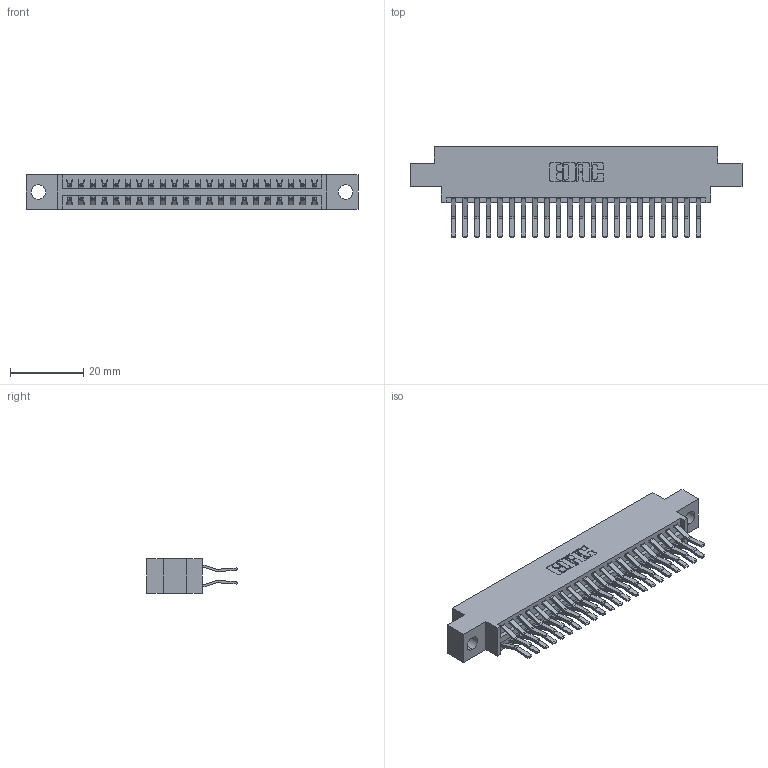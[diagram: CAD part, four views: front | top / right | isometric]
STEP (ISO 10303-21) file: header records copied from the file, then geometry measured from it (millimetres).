
FILE_DESCRIPTION (( 'STEP AP203' ), '1' );
FILE_NAME ('346-044-560-804.STEP', '2022-05-20T08:39:11', ( '' ), ( '' ), 'SwSTEP 2.0', 'SolidWorks 2020', '' );
FILE_SCHEMA (( 'CONFIG_CONTROL_DESIGN' ));
Length unit declared in the file: inch
Products named in the file (3): 346 Part_0.170 Offset - 0.156 Dia-TH; 346-044-560-804; 345-292-001_560 Tail
Assembly tree (45 placements, depth 2):
  346-044-560-804
    346 Part_0.170 Offset - 0.156 Dia-TH
    345-292-001_560 Tail  x44
Bounding box: 90.42 x 24.78 x 9.4 mm (x, y, z)
Volume: 8690 mm3; surface area: 12427.6 mm2
Topology: 45 solids, 45 shells, 2516 faces, 7461 edges, 4914 vertices
Faces by surface type: plane 1634, cylinder 882
Entity records: 17689 total; most frequent: CARTESIAN_POINT 2950, ORIENTED_EDGE 2882, DIRECTION 2653, EDGE_CURVE 1441, VECTOR 1217, LINE 1217, VERTEX_POINT 958, AXIS2_PLACEMENT_3D 718
